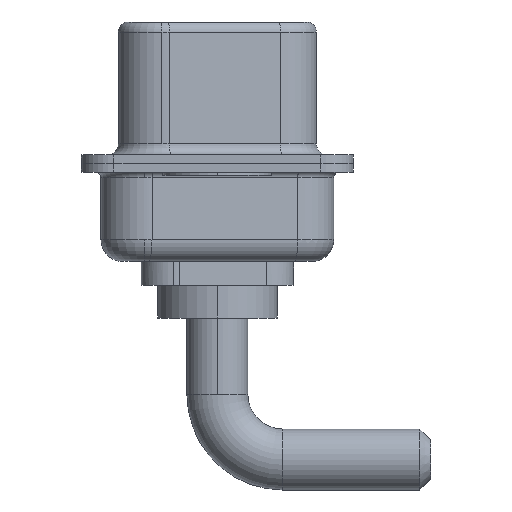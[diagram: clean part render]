
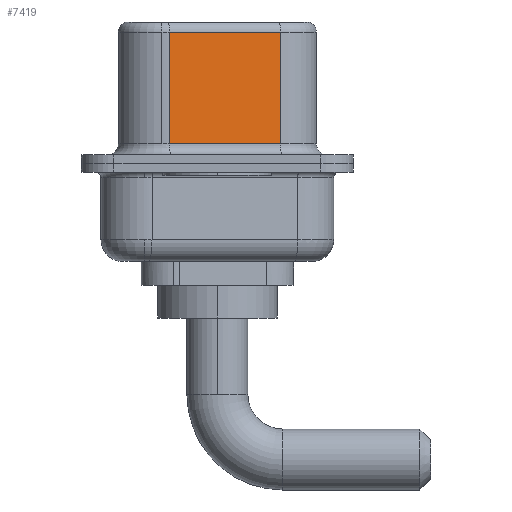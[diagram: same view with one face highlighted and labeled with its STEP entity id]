
A CAD part, left-side view. The second image highlights one B-rep face of the part: STEP entity #7419.
In plain terms, the highlighted planar face has unit normal (-0.985, -0.174, 0).
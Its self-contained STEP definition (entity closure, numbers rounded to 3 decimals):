
#316 = CARTESIAN_POINT ( 'NONE',  ( 4.555, -2.897, 6.52 ) ) ;
#420 = DIRECTION ( 'NONE',  ( -0.174, 0.985, 0. ) ) ;
#1111 = EDGE_CURVE ( 'NONE', #6048, #1565, #11247, .T. ) ;
#1142 = AXIS2_PLACEMENT_3D ( 'NONE', #3597, #7852, #420 ) ;
#1298 = DIRECTION ( 'NONE',  ( 0., 0., -1. ) ) ;
#1543 = FACE_OUTER_BOUND ( 'NONE', #6509, .T. ) ;
#1565 = VERTEX_POINT ( 'NONE', #13343 ) ;
#1568 = ORIENTED_EDGE ( 'NONE', *, *, #12784, .T. ) ;
#2155 = CARTESIAN_POINT ( 'NONE',  ( 3.655, 2.203, 6.52 ) ) ;
#2561 = DIRECTION ( 'NONE',  ( 0.174, -0.985, 0. ) ) ;
#3597 = CARTESIAN_POINT ( 'NONE',  ( 4.555, -2.897, 6.52 ) ) ;
#3674 = CARTESIAN_POINT ( 'NONE',  ( 3.655, 2.203, 6.02 ) ) ;
#4093 = DIRECTION ( 'NONE',  ( -0.174, 0.985, 0. ) ) ;
#4428 = CARTESIAN_POINT ( 'NONE',  ( 4.555, -2.897, 6.02 ) ) ;
#4491 = PLANE ( 'NONE',  #1142 ) ;
#4555 = VECTOR ( 'NONE', #2561, 1000. ) ;
#4606 = DIRECTION ( 'NONE',  ( 0., 0., -1. ) ) ;
#5165 = ORIENTED_EDGE ( 'NONE', *, *, #13115, .T. ) ;
#5990 = CARTESIAN_POINT ( 'NONE',  ( 4.555, -2.897, 0.9 ) ) ;
#6048 = VERTEX_POINT ( 'NONE', #7024 ) ;
#6509 = EDGE_LOOP ( 'NONE', ( #12352, #5165, #1568, #11965 ) ) ;
#7024 = CARTESIAN_POINT ( 'NONE',  ( 3.655, 2.203, 0.9 ) ) ;
#7322 = VERTEX_POINT ( 'NONE', #4428 ) ;
#7419 = ADVANCED_FACE ( 'NONE', ( #1543 ), #4491, .F. ) ;
#7852 = DIRECTION ( 'NONE',  ( 0.985, 0.174, 0. ) ) ;
#8163 = VERTEX_POINT ( 'NONE', #3674 ) ;
#8367 = LINE ( 'NONE', #13493, #12231 ) ;
#9519 = VECTOR ( 'NONE', #1298, 1000. ) ;
#9776 = LINE ( 'NONE', #2155, #9519 ) ;
#10764 = EDGE_CURVE ( 'NONE', #7322, #1565, #12120, .T. ) ;
#11247 = LINE ( 'NONE', #5990, #4555 ) ;
#11965 = ORIENTED_EDGE ( 'NONE', *, *, #1111, .T. ) ;
#12120 = LINE ( 'NONE', #316, #13101 ) ;
#12231 = VECTOR ( 'NONE', #4093, 1000. ) ;
#12352 = ORIENTED_EDGE ( 'NONE', *, *, #10764, .F. ) ;
#12784 = EDGE_CURVE ( 'NONE', #8163, #6048, #9776, .T. ) ;
#13101 = VECTOR ( 'NONE', #4606, 1000. ) ;
#13115 = EDGE_CURVE ( 'NONE', #7322, #8163, #8367, .T. ) ;
#13343 = CARTESIAN_POINT ( 'NONE',  ( 4.555, -2.897, 0.9 ) ) ;
#13493 = CARTESIAN_POINT ( 'NONE',  ( 4.555, -2.897, 6.02 ) ) ;
